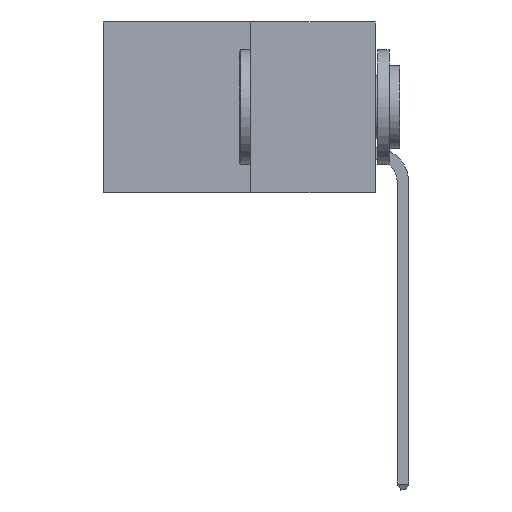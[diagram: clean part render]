
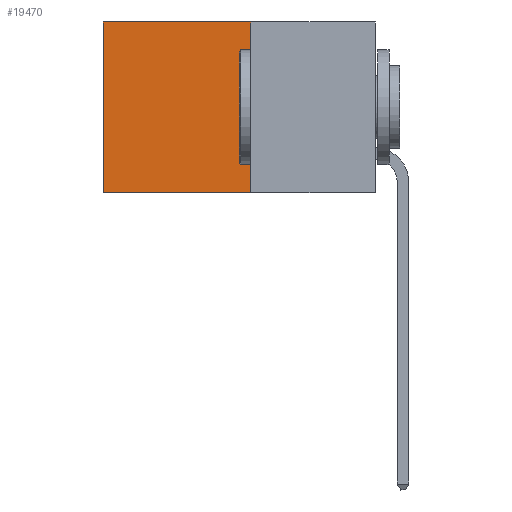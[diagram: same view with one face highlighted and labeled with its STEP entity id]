
A CAD part, left-side view. The second image highlights one B-rep face of the part: STEP entity #19470.
In plain terms, the highlighted planar face has unit normal (-1, 0, 0).
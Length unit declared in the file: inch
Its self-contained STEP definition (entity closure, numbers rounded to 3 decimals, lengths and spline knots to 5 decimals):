
#1785 = ORIENTED_EDGE ( 'NONE', *, *, #17529, .T. ) ;
#1909 = EDGE_LOOP ( 'NONE', ( #1785, #17300, #18899, #10292 ) ) ;
#2179 = CARTESIAN_POINT ( 'NONE',  ( 0.277, 0.27, -0.37 ) ) ;
#2698 = EDGE_CURVE ( 'NONE', #11787, #10461, #5527, .T. ) ;
#3334 = CARTESIAN_POINT ( 'NONE',  ( 0.277, 0.27, -0.37 ) ) ;
#3945 = CARTESIAN_POINT ( 'NONE',  ( 0.277, 0.59, -0.37 ) ) ;
#5527 = LINE ( 'NONE', #31158, #11751 ) ;
#6620 = DIRECTION ( 'NONE',  ( 0., 0., -1. ) ) ;
#7351 = PLANE ( 'NONE',  #20170 ) ;
#7431 = VECTOR ( 'NONE', #23016, 39.37008 ) ;
#8392 = VERTEX_POINT ( 'NONE', #3334 ) ;
#8771 = EDGE_CURVE ( 'NONE', #11787, #8392, #11874, .T. ) ;
#9440 = LINE ( 'NONE', #3945, #29147 ) ;
#10292 = ORIENTED_EDGE ( 'NONE', *, *, #2698, .T. ) ;
#10461 = VERTEX_POINT ( 'NONE', #29705 ) ;
#11504 = EDGE_CURVE ( 'NONE', #8392, #29612, #28058, .T. ) ;
#11751 = VECTOR ( 'NONE', #27533, 39.37008 ) ;
#11787 = VERTEX_POINT ( 'NONE', #27070 ) ;
#11874 = LINE ( 'NONE', #33182, #24739 ) ;
#12666 = DIRECTION ( 'NONE',  ( 1., 0., 0. ) ) ;
#17300 = ORIENTED_EDGE ( 'NONE', *, *, #11504, .F. ) ;
#17529 = EDGE_CURVE ( 'NONE', #10461, #29612, #9440, .T. ) ;
#18899 = ORIENTED_EDGE ( 'NONE', *, *, #8771, .F. ) ;
#19470 = ADVANCED_FACE ( 'NONE', ( #27035 ), #7351, .F. ) ;
#19864 = CARTESIAN_POINT ( 'NONE',  ( 0.277, 0.59, -0.37 ) ) ;
#20170 = AXIS2_PLACEMENT_3D ( 'NONE', #28040, #12666, #30525 ) ;
#23016 = DIRECTION ( 'NONE',  ( 0., 1., 0. ) ) ;
#23107 = DIRECTION ( 'NONE',  ( 0., 0., -1. ) ) ;
#24739 = VECTOR ( 'NONE', #23107, 39.37008 ) ;
#27035 = FACE_OUTER_BOUND ( 'NONE', #1909, .T. ) ;
#27070 = CARTESIAN_POINT ( 'NONE',  ( 0.277, 0.27, 0. ) ) ;
#27533 = DIRECTION ( 'NONE',  ( 0., 1., 0. ) ) ;
#28040 = CARTESIAN_POINT ( 'NONE',  ( 0.277, 0.27, -0.37 ) ) ;
#28058 = LINE ( 'NONE', #2179, #7431 ) ;
#29147 = VECTOR ( 'NONE', #6620, 39.37008 ) ;
#29612 = VERTEX_POINT ( 'NONE', #19864 ) ;
#29705 = CARTESIAN_POINT ( 'NONE',  ( 0.277, 0.59, 0. ) ) ;
#30525 = DIRECTION ( 'NONE',  ( 0., 0., -1. ) ) ;
#31158 = CARTESIAN_POINT ( 'NONE',  ( 0.277, 0.27, 0. ) ) ;
#33182 = CARTESIAN_POINT ( 'NONE',  ( 0.277, 0.27, -0.37 ) ) ;
